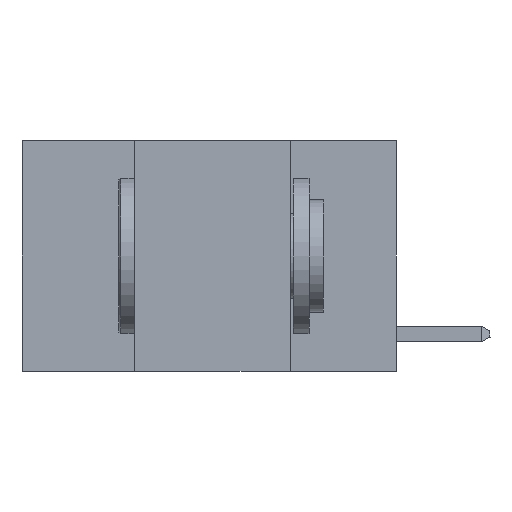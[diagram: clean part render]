
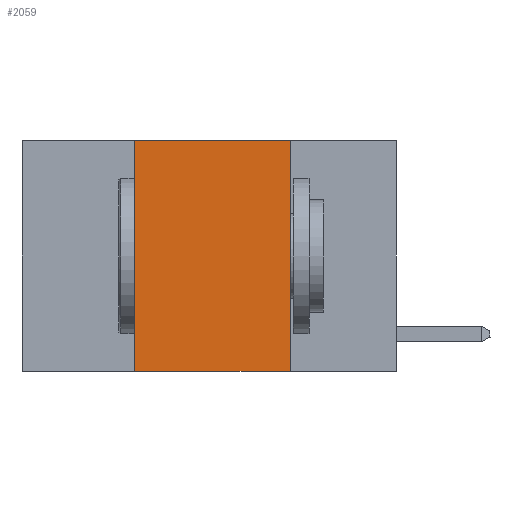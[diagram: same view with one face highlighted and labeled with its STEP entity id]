
A CAD part, left-side view. The second image highlights one B-rep face of the part: STEP entity #2059.
In plain terms, the highlighted planar face has unit normal (-1, 0, 0).
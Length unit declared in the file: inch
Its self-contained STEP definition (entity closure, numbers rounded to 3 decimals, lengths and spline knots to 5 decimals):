
#217 = CARTESIAN_POINT ( 'NONE',  ( 0., 0.42, -0.37 ) ) ;
#234 = EDGE_CURVE ( 'NONE', #8613, #2983, #5980, .T. ) ;
#852 = LINE ( 'NONE', #8049, #5639 ) ;
#1017 = CARTESIAN_POINT ( 'NONE',  ( 0., 0.42, 0. ) ) ;
#1944 = ORIENTED_EDGE ( 'NONE', *, *, #234, .F. ) ;
#2059 = ADVANCED_FACE ( 'NONE', ( #7914 ), #5865, .F. ) ;
#2121 = VERTEX_POINT ( 'NONE', #3931 ) ;
#2733 = DIRECTION ( 'NONE',  ( 1., 0., 0. ) ) ;
#2983 = VERTEX_POINT ( 'NONE', #7461 ) ;
#2992 = DIRECTION ( 'NONE',  ( 0., -1., 0. ) ) ;
#3732 = CARTESIAN_POINT ( 'NONE',  ( 0., 0.6, 0. ) ) ;
#3931 = CARTESIAN_POINT ( 'NONE',  ( 0., 0.42, 0. ) ) ;
#4144 = ORIENTED_EDGE ( 'NONE', *, *, #10107, .F. ) ;
#4731 = CARTESIAN_POINT ( 'NONE',  ( 0., 0.17, 0. ) ) ;
#5639 = VECTOR ( 'NONE', #2992, 39.37008 ) ;
#5865 = PLANE ( 'NONE',  #9589 ) ;
#5912 = DIRECTION ( 'NONE',  ( 0., 0., -1. ) ) ;
#5980 = LINE ( 'NONE', #4731, #9657 ) ;
#6288 = EDGE_CURVE ( 'NONE', #2121, #8613, #852, .T. ) ;
#6775 = DIRECTION ( 'NONE',  ( 0., 0., -1. ) ) ;
#7461 = CARTESIAN_POINT ( 'NONE',  ( 0., 0.17, -0.37 ) ) ;
#7829 = LINE ( 'NONE', #7904, #13056 ) ;
#7904 = CARTESIAN_POINT ( 'NONE',  ( 0., 0.6, -0.37 ) ) ;
#7914 = FACE_OUTER_BOUND ( 'NONE', #7989, .T. ) ;
#7989 = EDGE_LOOP ( 'NONE', ( #1944, #9950, #4144, #11472 ) ) ;
#8049 = CARTESIAN_POINT ( 'NONE',  ( 0., 0.6, 0. ) ) ;
#8613 = VERTEX_POINT ( 'NONE', #9072 ) ;
#9072 = CARTESIAN_POINT ( 'NONE',  ( 0., 0.17, 0. ) ) ;
#9589 = AXIS2_PLACEMENT_3D ( 'NONE', #3732, #2733, #6775 ) ;
#9657 = VECTOR ( 'NONE', #5912, 39.37008 ) ;
#9872 = VERTEX_POINT ( 'NONE', #217 ) ;
#9950 = ORIENTED_EDGE ( 'NONE', *, *, #6288, .F. ) ;
#9995 = DIRECTION ( 'NONE',  ( 0., -1., 0. ) ) ;
#10107 = EDGE_CURVE ( 'NONE', #9872, #2121, #10152, .T. ) ;
#10152 = LINE ( 'NONE', #1017, #11247 ) ;
#11247 = VECTOR ( 'NONE', #11366, 39.37008 ) ;
#11366 = DIRECTION ( 'NONE',  ( 0., 0., 1. ) ) ;
#11472 = ORIENTED_EDGE ( 'NONE', *, *, #12904, .T. ) ;
#12904 = EDGE_CURVE ( 'NONE', #9872, #2983, #7829, .T. ) ;
#13056 = VECTOR ( 'NONE', #9995, 39.37008 ) ;
